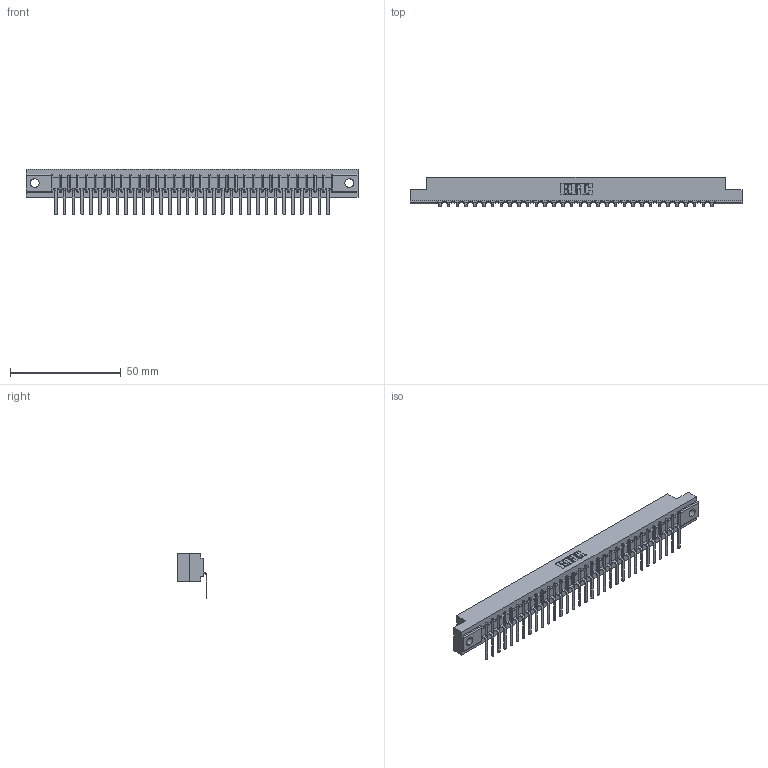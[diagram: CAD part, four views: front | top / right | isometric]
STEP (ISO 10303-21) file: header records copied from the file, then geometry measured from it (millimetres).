
FILE_DESCRIPTION (( 'STEP AP203' ), '1' );
FILE_NAME ('357-032-457-102.STEP', '2020-10-02T06:24:54', ( '' ), ( '' ), 'SwSTEP 2.0', 'SolidWorks 2020', '' );
FILE_SCHEMA (( 'CONFIG_CONTROL_DESIGN' ));
Length unit declared in the file: inch
Products named in the file (3): 307-290-002_557; 307 Part_.128 Dia Mounting Holes; 357-032-457-102
Assembly tree (33 placements, depth 2):
  357-032-457-102
    307 Part_.128 Dia Mounting Holes
    307-290-002_557  x32
Bounding box: 149.81 x 13.32 x 20.66 mm (x, y, z)
Volume: 15955.4 mm3; surface area: 20207.5 mm2
Topology: 33 solids, 33 shells, 2647 faces, 8131 edges, 5330 vertices
Faces by surface type: plane 1574, cylinder 1007, sphere 66
Entity records: 29522 total; most frequent: CARTESIAN_POINT 4980, ORIENTED_EDGE 4970, DIRECTION 4843, EDGE_CURVE 2485, LINE 1897, VECTOR 1897, VERTEX_POINT 1610, AXIS2_PLACEMENT_3D 1473
